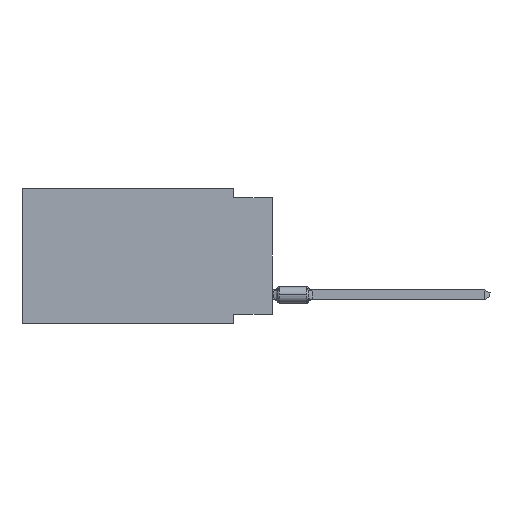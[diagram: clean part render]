
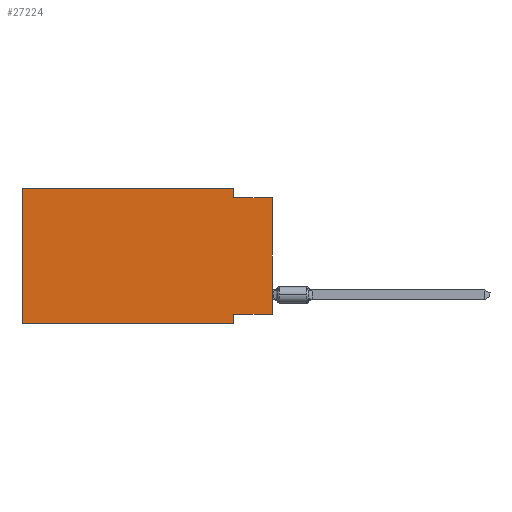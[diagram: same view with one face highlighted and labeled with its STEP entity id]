
A CAD part, left-side view. The second image highlights one B-rep face of the part: STEP entity #27224.
In plain terms, the highlighted planar face has unit normal (-1, 0, 0).
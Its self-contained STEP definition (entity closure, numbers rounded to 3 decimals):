
#321 = VERTEX_POINT ( 'NONE', #33669 ) ;
#494 = ORIENTED_EDGE ( 'NONE', *, *, #32351, .F. ) ;
#2128 = VECTOR ( 'NONE', #29133, 1000. ) ;
#2353 = EDGE_CURVE ( 'NONE', #26337, #30850, #33045, .T. ) ;
#2381 = LINE ( 'NONE', #7542, #13465 ) ;
#3281 = CARTESIAN_POINT ( 'NONE',  ( 0., 0., -8.255 ) ) ;
#3688 = VERTEX_POINT ( 'NONE', #39410 ) ;
#7542 = CARTESIAN_POINT ( 'NONE',  ( 0., 16.383, 0. ) ) ;
#7816 = EDGE_CURVE ( 'NONE', #10043, #47322, #20591, .T. ) ;
#8174 = AXIS2_PLACEMENT_3D ( 'NONE', #44628, #41591, #26251 ) ;
#9746 = ORIENTED_EDGE ( 'NONE', *, *, #22469, .F. ) ;
#9781 = VECTOR ( 'NONE', #22606, 1000. ) ;
#9908 = VERTEX_POINT ( 'NONE', #22649 ) ;
#10043 = VERTEX_POINT ( 'NONE', #39465 ) ;
#10355 = DIRECTION ( 'NONE',  ( 0., 1., 0. ) ) ;
#10428 = PLANE ( 'NONE',  #8174 ) ;
#13465 = VECTOR ( 'NONE', #26127, 1000. ) ;
#13811 = CARTESIAN_POINT ( 'NONE',  ( 0., 0., 0. ) ) ;
#14453 = FACE_OUTER_BOUND ( 'NONE', #22592, .T. ) ;
#14871 = VECTOR ( 'NONE', #25633, 1000. ) ;
#15825 = CARTESIAN_POINT ( 'NONE',  ( 0., 2.54, 0. ) ) ;
#15910 = ORIENTED_EDGE ( 'NONE', *, *, #7816, .F. ) ;
#17476 = DIRECTION ( 'NONE',  ( 0., 0., -1. ) ) ;
#17600 = VECTOR ( 'NONE', #23620, 1000. ) ;
#20149 = CARTESIAN_POINT ( 'NONE',  ( 0., 2.54, -8.89 ) ) ;
#20591 = LINE ( 'NONE', #15825, #17600 ) ;
#21744 = CARTESIAN_POINT ( 'NONE',  ( 0., 2.54, -8.89 ) ) ;
#22469 = EDGE_CURVE ( 'NONE', #3688, #321, #2381, .T. ) ;
#22592 = EDGE_LOOP ( 'NONE', ( #27097, #25659, #15910, #494, #9746, #28124, #48782, #41448 ) ) ;
#22606 = DIRECTION ( 'NONE',  ( 0., -1., 0. ) ) ;
#22649 = CARTESIAN_POINT ( 'NONE',  ( 0., 0., -0.635 ) ) ;
#23361 = CARTESIAN_POINT ( 'NONE',  ( 0., 16.383, -8.89 ) ) ;
#23620 = DIRECTION ( 'NONE',  ( 0., 0., -1. ) ) ;
#24076 = VECTOR ( 'NONE', #42533, 1000. ) ;
#24907 = CARTESIAN_POINT ( 'NONE',  ( 0., 16.383, 0. ) ) ;
#25633 = DIRECTION ( 'NONE',  ( 0., -1., 0. ) ) ;
#25659 = ORIENTED_EDGE ( 'NONE', *, *, #49251, .F. ) ;
#25926 = LINE ( 'NONE', #30190, #36576 ) ;
#26127 = DIRECTION ( 'NONE',  ( 0., 0., 1. ) ) ;
#26251 = DIRECTION ( 'NONE',  ( 0., 0., -1. ) ) ;
#26337 = VERTEX_POINT ( 'NONE', #42865 ) ;
#27097 = ORIENTED_EDGE ( 'NONE', *, *, #42506, .T. ) ;
#27224 = ADVANCED_FACE ( 'NONE', ( #14453 ), #10428, .F. ) ;
#27423 = CARTESIAN_POINT ( 'NONE',  ( 0., 0., -0.635 ) ) ;
#28124 = ORIENTED_EDGE ( 'NONE', *, *, #36313, .T. ) ;
#29133 = DIRECTION ( 'NONE',  ( 0., 0., 1. ) ) ;
#30062 = VERTEX_POINT ( 'NONE', #3281 ) ;
#30190 = CARTESIAN_POINT ( 'NONE',  ( 0., 0., -8.255 ) ) ;
#30850 = VERTEX_POINT ( 'NONE', #20149 ) ;
#32351 = EDGE_CURVE ( 'NONE', #321, #10043, #44020, .T. ) ;
#32898 = EDGE_CURVE ( 'NONE', #30062, #26337, #25926, .T. ) ;
#33045 = LINE ( 'NONE', #21744, #36551 ) ;
#33048 = CARTESIAN_POINT ( 'NONE',  ( 0., 2.54, -0.635 ) ) ;
#33669 = CARTESIAN_POINT ( 'NONE',  ( 0., 16.383, 0. ) ) ;
#36313 = EDGE_CURVE ( 'NONE', #3688, #30850, #45735, .T. ) ;
#36551 = VECTOR ( 'NONE', #17476, 1000. ) ;
#36576 = VECTOR ( 'NONE', #10355, 1000. ) ;
#39410 = CARTESIAN_POINT ( 'NONE',  ( 0., 16.383, -8.89 ) ) ;
#39465 = CARTESIAN_POINT ( 'NONE',  ( 0., 2.54, 0. ) ) ;
#41448 = ORIENTED_EDGE ( 'NONE', *, *, #32898, .F. ) ;
#41591 = DIRECTION ( 'NONE',  ( 1., 0., 0. ) ) ;
#42506 = EDGE_CURVE ( 'NONE', #30062, #9908, #48247, .T. ) ;
#42533 = DIRECTION ( 'NONE',  ( 0., -1., 0. ) ) ;
#42865 = CARTESIAN_POINT ( 'NONE',  ( 0., 2.54, -8.255 ) ) ;
#44020 = LINE ( 'NONE', #24907, #14871 ) ;
#44628 = CARTESIAN_POINT ( 'NONE',  ( 0., 16.383, 0. ) ) ;
#45735 = LINE ( 'NONE', #23361, #9781 ) ;
#47296 = LINE ( 'NONE', #27423, #24076 ) ;
#47322 = VERTEX_POINT ( 'NONE', #33048 ) ;
#48247 = LINE ( 'NONE', #13811, #2128 ) ;
#48782 = ORIENTED_EDGE ( 'NONE', *, *, #2353, .F. ) ;
#49251 = EDGE_CURVE ( 'NONE', #47322, #9908, #47296, .T. ) ;
